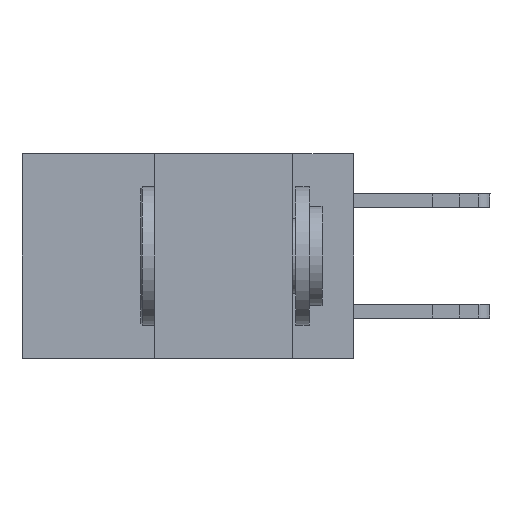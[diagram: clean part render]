
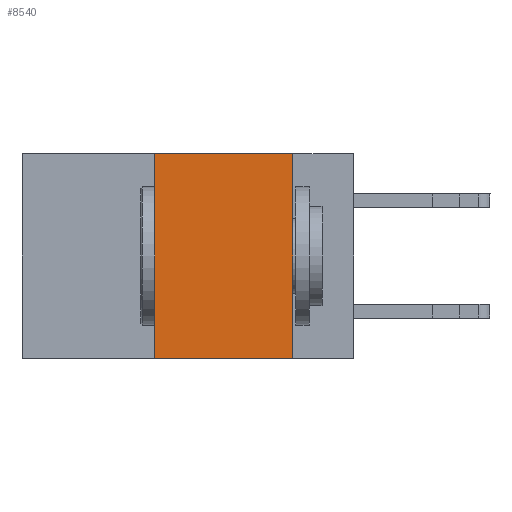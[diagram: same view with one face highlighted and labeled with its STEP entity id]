
A CAD part, left-side view. The second image highlights one B-rep face of the part: STEP entity #8540.
In plain terms, the highlighted planar face has unit normal (-1, 0, 0).
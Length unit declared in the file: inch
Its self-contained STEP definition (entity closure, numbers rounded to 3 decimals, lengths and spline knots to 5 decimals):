
#27 = VECTOR ( 'NONE', #28796, 39.37008 ) ;
#250 = CARTESIAN_POINT ( 'NONE',  ( 0., 0.6, 0. ) ) ;
#926 = LINE ( 'NONE', #2195, #6339 ) ;
#1870 = CARTESIAN_POINT ( 'NONE',  ( 0., 0.36, 0. ) ) ;
#2195 = CARTESIAN_POINT ( 'NONE',  ( 0., 0.6, 0. ) ) ;
#2330 = VERTEX_POINT ( 'NONE', #18051 ) ;
#6339 = VECTOR ( 'NONE', #19539, 39.37008 ) ;
#6391 = VERTEX_POINT ( 'NONE', #29680 ) ;
#7762 = EDGE_CURVE ( 'NONE', #17738, #30617, #14572, .T. ) ;
#7924 = ORIENTED_EDGE ( 'NONE', *, *, #30695, .F. ) ;
#8024 = LINE ( 'NONE', #12057, #27 ) ;
#8540 = ADVANCED_FACE ( 'NONE', ( #24914 ), #29426, .F. ) ;
#8854 = VECTOR ( 'NONE', #18994, 39.37008 ) ;
#9567 = ORIENTED_EDGE ( 'NONE', *, *, #14975, .F. ) ;
#12057 = CARTESIAN_POINT ( 'NONE',  ( 0., 0.11, 0. ) ) ;
#12186 = EDGE_LOOP ( 'NONE', ( #9567, #7924, #26665, #17423 ) ) ;
#12366 = DIRECTION ( 'NONE',  ( 1., 0., 0. ) ) ;
#13082 = CARTESIAN_POINT ( 'NONE',  ( 0., 0.36, 0. ) ) ;
#13449 = VECTOR ( 'NONE', #17307, 39.37008 ) ;
#14391 = EDGE_CURVE ( 'NONE', #17738, #6391, #27632, .T. ) ;
#14572 = LINE ( 'NONE', #1870, #8854 ) ;
#14704 = DIRECTION ( 'NONE',  ( 0., 0., -1. ) ) ;
#14975 = EDGE_CURVE ( 'NONE', #2330, #6391, #8024, .T. ) ;
#17307 = DIRECTION ( 'NONE',  ( 0., -1., 0. ) ) ;
#17423 = ORIENTED_EDGE ( 'NONE', *, *, #14391, .T. ) ;
#17461 = CARTESIAN_POINT ( 'NONE',  ( 0., 0.36, -0.37 ) ) ;
#17738 = VERTEX_POINT ( 'NONE', #17461 ) ;
#18051 = CARTESIAN_POINT ( 'NONE',  ( 0., 0.11, 0. ) ) ;
#18994 = DIRECTION ( 'NONE',  ( 0., 0., 1. ) ) ;
#19539 = DIRECTION ( 'NONE',  ( 0., -1., 0. ) ) ;
#23631 = AXIS2_PLACEMENT_3D ( 'NONE', #250, #12366, #14704 ) ;
#24914 = FACE_OUTER_BOUND ( 'NONE', #12186, .T. ) ;
#26665 = ORIENTED_EDGE ( 'NONE', *, *, #7762, .F. ) ;
#27632 = LINE ( 'NONE', #29456, #13449 ) ;
#28796 = DIRECTION ( 'NONE',  ( 0., 0., -1. ) ) ;
#29426 = PLANE ( 'NONE',  #23631 ) ;
#29456 = CARTESIAN_POINT ( 'NONE',  ( 0., 0.6, -0.37 ) ) ;
#29680 = CARTESIAN_POINT ( 'NONE',  ( 0., 0.11, -0.37 ) ) ;
#30617 = VERTEX_POINT ( 'NONE', #13082 ) ;
#30695 = EDGE_CURVE ( 'NONE', #30617, #2330, #926, .T. ) ;
